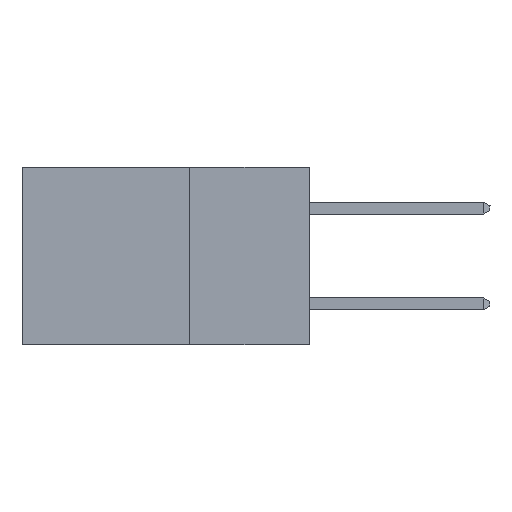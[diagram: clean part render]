
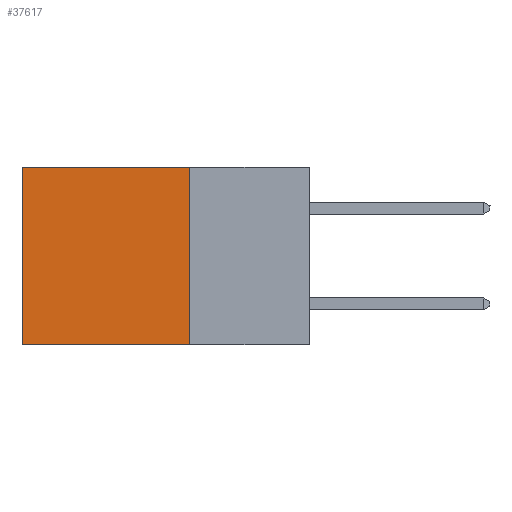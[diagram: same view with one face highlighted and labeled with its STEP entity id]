
A CAD part, left-side view. The second image highlights one B-rep face of the part: STEP entity #37617.
In plain terms, the highlighted planar face has unit normal (-1, 0, 0).
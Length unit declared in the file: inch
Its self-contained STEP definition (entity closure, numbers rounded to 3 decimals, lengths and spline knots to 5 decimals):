
#440 = LINE ( 'NONE', #28579, #33928 ) ;
#637 = DIRECTION ( 'NONE',  ( 0., 1., 0. ) ) ;
#2292 = LINE ( 'NONE', #5575, #34122 ) ;
#3973 = EDGE_CURVE ( 'NONE', #39435, #12738, #10321, .T. ) ;
#5287 = AXIS2_PLACEMENT_3D ( 'NONE', #41998, #19065, #35658 ) ;
#5575 = CARTESIAN_POINT ( 'NONE',  ( 0.2875, 0.6, 0. ) ) ;
#8570 = FACE_OUTER_BOUND ( 'NONE', #18016, .T. ) ;
#10321 = LINE ( 'NONE', #24222, #10864 ) ;
#10864 = VECTOR ( 'NONE', #637, 39.37008 ) ;
#10881 = EDGE_CURVE ( 'NONE', #16128, #39885, #42058, .T. ) ;
#12441 = CARTESIAN_POINT ( 'NONE',  ( 0.2875, 0.6, 0. ) ) ;
#12457 = PLANE ( 'NONE',  #5287 ) ;
#12738 = VERTEX_POINT ( 'NONE', #28286 ) ;
#16128 = VERTEX_POINT ( 'NONE', #16482 ) ;
#16482 = CARTESIAN_POINT ( 'NONE',  ( 0.2875, 0.25, 0. ) ) ;
#18016 = EDGE_LOOP ( 'NONE', ( #19885, #28297, #24361, #27558 ) ) ;
#19065 = DIRECTION ( 'NONE',  ( 1., 0., 0. ) ) ;
#19885 = ORIENTED_EDGE ( 'NONE', *, *, #26556, .T. ) ;
#20084 = VECTOR ( 'NONE', #20866, 39.37008 ) ;
#20866 = DIRECTION ( 'NONE',  ( 0., 1., 0. ) ) ;
#21689 = CARTESIAN_POINT ( 'NONE',  ( 0.2875, 0.25, -0.37 ) ) ;
#23800 = CARTESIAN_POINT ( 'NONE',  ( 0.2875, 0.25, 0. ) ) ;
#24222 = CARTESIAN_POINT ( 'NONE',  ( 0.2875, 0.25, -0.37 ) ) ;
#24361 = ORIENTED_EDGE ( 'NONE', *, *, #42278, .F. ) ;
#26556 = EDGE_CURVE ( 'NONE', #39885, #12738, #2292, .T. ) ;
#27558 = ORIENTED_EDGE ( 'NONE', *, *, #10881, .T. ) ;
#28286 = CARTESIAN_POINT ( 'NONE',  ( 0.2875, 0.6, -0.37 ) ) ;
#28297 = ORIENTED_EDGE ( 'NONE', *, *, #3973, .F. ) ;
#28579 = CARTESIAN_POINT ( 'NONE',  ( 0.2875, 0.25, 0. ) ) ;
#32439 = DIRECTION ( 'NONE',  ( 0., 0., -1. ) ) ;
#33928 = VECTOR ( 'NONE', #35812, 39.37008 ) ;
#34122 = VECTOR ( 'NONE', #32439, 39.37008 ) ;
#35658 = DIRECTION ( 'NONE',  ( 0., 0., -1. ) ) ;
#35812 = DIRECTION ( 'NONE',  ( 0., 0., -1. ) ) ;
#37617 = ADVANCED_FACE ( 'NONE', ( #8570 ), #12457, .F. ) ;
#39435 = VERTEX_POINT ( 'NONE', #21689 ) ;
#39885 = VERTEX_POINT ( 'NONE', #12441 ) ;
#41998 = CARTESIAN_POINT ( 'NONE',  ( 0.2875, 0.25, 0. ) ) ;
#42058 = LINE ( 'NONE', #23800, #20084 ) ;
#42278 = EDGE_CURVE ( 'NONE', #16128, #39435, #440, .T. ) ;
